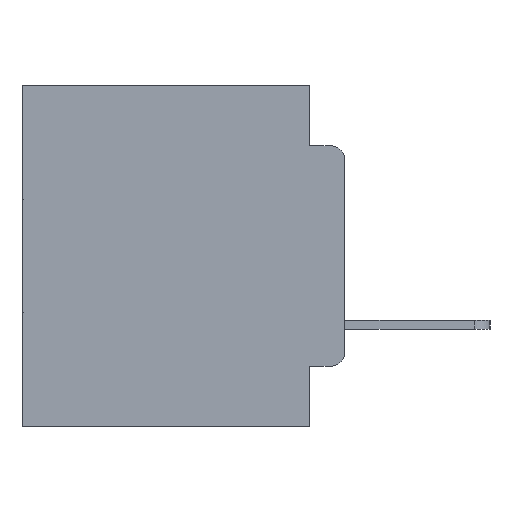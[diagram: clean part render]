
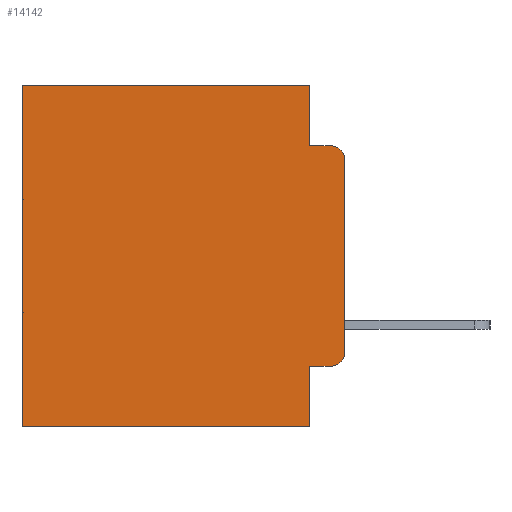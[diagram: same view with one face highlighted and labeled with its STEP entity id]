
A CAD part, left-side view. The second image highlights one B-rep face of the part: STEP entity #14142.
In plain terms, the highlighted planar face has unit normal (-1, 0, 0).
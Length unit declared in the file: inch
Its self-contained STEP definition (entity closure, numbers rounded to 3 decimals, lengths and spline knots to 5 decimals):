
#107 = VECTOR ( 'NONE', #26889, 39.37008 ) ;
#563 = VERTEX_POINT ( 'NONE', #22806 ) ;
#718 = EDGE_CURVE ( 'NONE', #563, #20670, #2765, .T. ) ;
#950 = VERTEX_POINT ( 'NONE', #10387 ) ;
#1289 = EDGE_CURVE ( 'NONE', #28837, #950, #27098, .T. ) ;
#2252 = CARTESIAN_POINT ( 'NONE',  ( 0.298, 0.051, -0.4115 ) ) ;
#2296 = VERTEX_POINT ( 'NONE', #22338 ) ;
#2557 = LINE ( 'NONE', #8139, #15133 ) ;
#2765 = CIRCLE ( 'NONE', #21238, 0.02 ) ;
#3282 = CARTESIAN_POINT ( 'NONE',  ( 0.298, 0.051, -0.0885 ) ) ;
#4330 = EDGE_CURVE ( 'NONE', #25748, #20670, #26949, .T. ) ;
#4404 = VERTEX_POINT ( 'NONE', #17833 ) ;
#4615 = EDGE_CURVE ( 'NONE', #18667, #563, #24553, .T. ) ;
#4668 = CARTESIAN_POINT ( 'NONE',  ( 0.298, 0.02, -0.3915 ) ) ;
#5001 = DIRECTION ( 'NONE',  ( 0., 0., -1. ) ) ;
#5317 = DIRECTION ( 'NONE',  ( -1., 0., 0. ) ) ;
#5333 = EDGE_LOOP ( 'NONE', ( #29280, #23196, #23898, #7282, #16210, #22142, #29993, #25599, #17322, #11648 ) ) ;
#6474 = VECTOR ( 'NONE', #30299, 39.37008 ) ;
#6621 = DIRECTION ( 'NONE',  ( 0., 0., -1. ) ) ;
#7282 = ORIENTED_EDGE ( 'NONE', *, *, #24080, .F. ) ;
#7430 = DIRECTION ( 'NONE',  ( 0., 0., -1. ) ) ;
#8139 = CARTESIAN_POINT ( 'NONE',  ( 0.298, 0., -0.5 ) ) ;
#8832 = CARTESIAN_POINT ( 'NONE',  ( 0.298, 0.051, -0.0885 ) ) ;
#9232 = DIRECTION ( 'NONE',  ( -1., 0., 0. ) ) ;
#9702 = CARTESIAN_POINT ( 'NONE',  ( 0.298, 0., -0.3915 ) ) ;
#9722 = CARTESIAN_POINT ( 'NONE',  ( 0.298, 0.051, -0.4115 ) ) ;
#10387 = CARTESIAN_POINT ( 'NONE',  ( 0.298, 0.473, -0.5 ) ) ;
#10425 = VECTOR ( 'NONE', #7430, 39.37008 ) ;
#10551 = EDGE_CURVE ( 'NONE', #14001, #2296, #18149, .T. ) ;
#11143 = EDGE_CURVE ( 'NONE', #25748, #2296, #24353, .T. ) ;
#11186 = LINE ( 'NONE', #19471, #10425 ) ;
#11648 = ORIENTED_EDGE ( 'NONE', *, *, #718, .T. ) ;
#12244 = CARTESIAN_POINT ( 'NONE',  ( 0.298, 0., 0. ) ) ;
#12770 = EDGE_CURVE ( 'NONE', #4404, #28837, #27947, .T. ) ;
#12885 = CARTESIAN_POINT ( 'NONE',  ( 0.298, 0.473, 0. ) ) ;
#13760 = DIRECTION ( 'NONE',  ( 0., -1., 0. ) ) ;
#13887 = AXIS2_PLACEMENT_3D ( 'NONE', #23254, #9232, #25449 ) ;
#14001 = VERTEX_POINT ( 'NONE', #3282 ) ;
#14142 = ADVANCED_FACE ( 'NONE', ( #22405 ), #29658, .F. ) ;
#14383 = CARTESIAN_POINT ( 'NONE',  ( 0.298, 0.473, 0. ) ) ;
#15101 = VECTOR ( 'NONE', #28597, 39.37008 ) ;
#15133 = VECTOR ( 'NONE', #24525, 39.37008 ) ;
#15999 = VECTOR ( 'NONE', #17817, 39.37008 ) ;
#16210 = ORIENTED_EDGE ( 'NONE', *, *, #12770, .T. ) ;
#17322 = ORIENTED_EDGE ( 'NONE', *, *, #4615, .T. ) ;
#17817 = DIRECTION ( 'NONE',  ( 0., 0., -1. ) ) ;
#17833 = CARTESIAN_POINT ( 'NONE',  ( 0.298, 0.051, 0. ) ) ;
#18149 = LINE ( 'NONE', #8832, #23367 ) ;
#18158 = CARTESIAN_POINT ( 'NONE',  ( 0.298, 0., 0. ) ) ;
#18667 = VERTEX_POINT ( 'NONE', #9722 ) ;
#19471 = CARTESIAN_POINT ( 'NONE',  ( 0.298, 0.051, 0. ) ) ;
#19773 = LINE ( 'NONE', #24715, #107 ) ;
#20670 = VERTEX_POINT ( 'NONE', #9702 ) ;
#20984 = DIRECTION ( 'NONE',  ( 1., 0., 0. ) ) ;
#21238 = AXIS2_PLACEMENT_3D ( 'NONE', #4668, #5317, #5001 ) ;
#22142 = ORIENTED_EDGE ( 'NONE', *, *, #1289, .T. ) ;
#22143 = VECTOR ( 'NONE', #23676, 39.37008 ) ;
#22338 = CARTESIAN_POINT ( 'NONE',  ( 0.298, 0.02, -0.0885 ) ) ;
#22405 = FACE_OUTER_BOUND ( 'NONE', #5333, .T. ) ;
#22806 = CARTESIAN_POINT ( 'NONE',  ( 0.298, 0.02, -0.4115 ) ) ;
#22836 = VERTEX_POINT ( 'NONE', #24726 ) ;
#23196 = ORIENTED_EDGE ( 'NONE', *, *, #11143, .T. ) ;
#23254 = CARTESIAN_POINT ( 'NONE',  ( 0.298, 0.02, -0.1085 ) ) ;
#23367 = VECTOR ( 'NONE', #13760, 39.37008 ) ;
#23676 = DIRECTION ( 'NONE',  ( 0., 1., 0. ) ) ;
#23898 = ORIENTED_EDGE ( 'NONE', *, *, #10551, .F. ) ;
#24080 = EDGE_CURVE ( 'NONE', #4404, #14001, #11186, .T. ) ;
#24353 = CIRCLE ( 'NONE', #13887, 0.02 ) ;
#24525 = DIRECTION ( 'NONE',  ( 0., 1., 0. ) ) ;
#24553 = LINE ( 'NONE', #2252, #6474 ) ;
#24715 = CARTESIAN_POINT ( 'NONE',  ( 0.298, 0.051, 0. ) ) ;
#24726 = CARTESIAN_POINT ( 'NONE',  ( 0.298, 0.051, -0.5 ) ) ;
#25449 = DIRECTION ( 'NONE',  ( 0., 0., -1. ) ) ;
#25599 = ORIENTED_EDGE ( 'NONE', *, *, #29340, .F. ) ;
#25748 = VERTEX_POINT ( 'NONE', #26820 ) ;
#26820 = CARTESIAN_POINT ( 'NONE',  ( 0.298, 0., -0.1085 ) ) ;
#26889 = DIRECTION ( 'NONE',  ( 0., 0., -1. ) ) ;
#26949 = LINE ( 'NONE', #18158, #15101 ) ;
#27098 = LINE ( 'NONE', #12885, #15999 ) ;
#27394 = CARTESIAN_POINT ( 'NONE',  ( 0.298, 0., 0. ) ) ;
#27947 = LINE ( 'NONE', #12244, #22143 ) ;
#27996 = AXIS2_PLACEMENT_3D ( 'NONE', #27394, #20984, #6621 ) ;
#28597 = DIRECTION ( 'NONE',  ( 0., 0., -1. ) ) ;
#28837 = VERTEX_POINT ( 'NONE', #14383 ) ;
#29258 = EDGE_CURVE ( 'NONE', #22836, #950, #2557, .T. ) ;
#29280 = ORIENTED_EDGE ( 'NONE', *, *, #4330, .F. ) ;
#29340 = EDGE_CURVE ( 'NONE', #18667, #22836, #19773, .T. ) ;
#29658 = PLANE ( 'NONE',  #27996 ) ;
#29993 = ORIENTED_EDGE ( 'NONE', *, *, #29258, .F. ) ;
#30299 = DIRECTION ( 'NONE',  ( 0., -1., 0. ) ) ;
